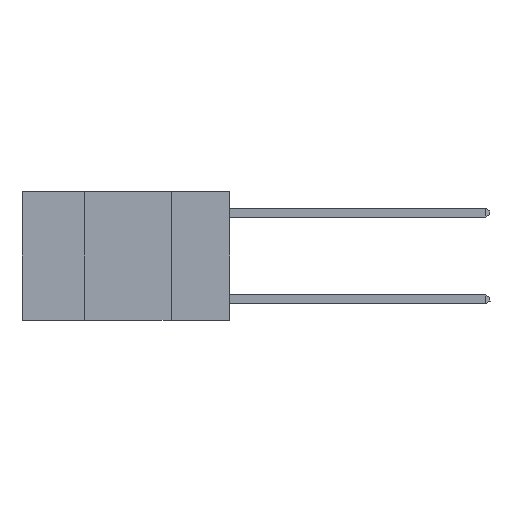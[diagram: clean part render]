
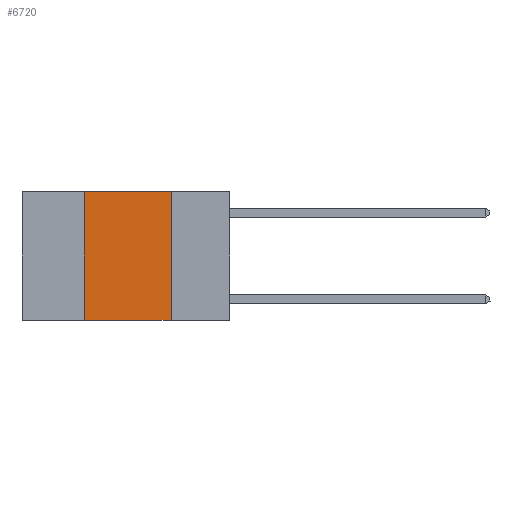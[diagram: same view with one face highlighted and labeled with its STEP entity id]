
A CAD part, left-side view. The second image highlights one B-rep face of the part: STEP entity #6720.
In plain terms, the highlighted planar face has unit normal (-1, 0, 0).
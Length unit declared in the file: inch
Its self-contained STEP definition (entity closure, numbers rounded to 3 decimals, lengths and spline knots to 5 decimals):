
#1017 = CARTESIAN_POINT ( 'NONE',  ( 0., 0.42, 0. ) ) ;
#1483 = EDGE_CURVE ( 'NONE', #2685, #5664, #3077, .T. ) ;
#2685 = VERTEX_POINT ( 'NONE', #17146 ) ;
#2949 = VECTOR ( 'NONE', #7805, 39.37008 ) ;
#3077 = LINE ( 'NONE', #10713, #22798 ) ;
#3774 = EDGE_CURVE ( 'NONE', #18727, #25497, #7813, .T. ) ;
#3938 = EDGE_CURVE ( 'NONE', #25497, #2685, #8117, .T. ) ;
#5664 = VERTEX_POINT ( 'NONE', #12458 ) ;
#6010 = EDGE_LOOP ( 'NONE', ( #20229, #8498, #14658, #16112 ) ) ;
#6406 = CARTESIAN_POINT ( 'NONE',  ( 0., 0.6, 0. ) ) ;
#6720 = ADVANCED_FACE ( 'NONE', ( #19265 ), #18211, .F. ) ;
#7805 = DIRECTION ( 'NONE',  ( 0., 0., 1. ) ) ;
#7813 = LINE ( 'NONE', #17585, #2949 ) ;
#8117 = LINE ( 'NONE', #10589, #12834 ) ;
#8489 = DIRECTION ( 'NONE',  ( 0., 0., -1. ) ) ;
#8498 = ORIENTED_EDGE ( 'NONE', *, *, #3938, .F. ) ;
#8813 = CARTESIAN_POINT ( 'NONE',  ( 0., 0.42, -0.37 ) ) ;
#10589 = CARTESIAN_POINT ( 'NONE',  ( 0., 0.6, 0. ) ) ;
#10713 = CARTESIAN_POINT ( 'NONE',  ( 0., 0.17, 0. ) ) ;
#12458 = CARTESIAN_POINT ( 'NONE',  ( 0., 0.17, -0.37 ) ) ;
#12562 = DIRECTION ( 'NONE',  ( 0., -1., 0. ) ) ;
#12834 = VECTOR ( 'NONE', #12562, 39.37008 ) ;
#14658 = ORIENTED_EDGE ( 'NONE', *, *, #3774, .F. ) ;
#15406 = EDGE_CURVE ( 'NONE', #18727, #5664, #15995, .T. ) ;
#15995 = LINE ( 'NONE', #22441, #22997 ) ;
#16112 = ORIENTED_EDGE ( 'NONE', *, *, #15406, .T. ) ;
#17146 = CARTESIAN_POINT ( 'NONE',  ( 0., 0.17, 0. ) ) ;
#17585 = CARTESIAN_POINT ( 'NONE',  ( 0., 0.42, 0. ) ) ;
#18211 = PLANE ( 'NONE',  #23781 ) ;
#18727 = VERTEX_POINT ( 'NONE', #8813 ) ;
#19265 = FACE_OUTER_BOUND ( 'NONE', #6010, .T. ) ;
#20155 = DIRECTION ( 'NONE',  ( 1., 0., 0. ) ) ;
#20229 = ORIENTED_EDGE ( 'NONE', *, *, #1483, .F. ) ;
#20380 = DIRECTION ( 'NONE',  ( 0., 0., -1. ) ) ;
#22441 = CARTESIAN_POINT ( 'NONE',  ( 0., 0.6, -0.37 ) ) ;
#22798 = VECTOR ( 'NONE', #20380, 39.37008 ) ;
#22997 = VECTOR ( 'NONE', #24316, 39.37008 ) ;
#23781 = AXIS2_PLACEMENT_3D ( 'NONE', #6406, #20155, #8489 ) ;
#24316 = DIRECTION ( 'NONE',  ( 0., -1., 0. ) ) ;
#25497 = VERTEX_POINT ( 'NONE', #1017 ) ;
